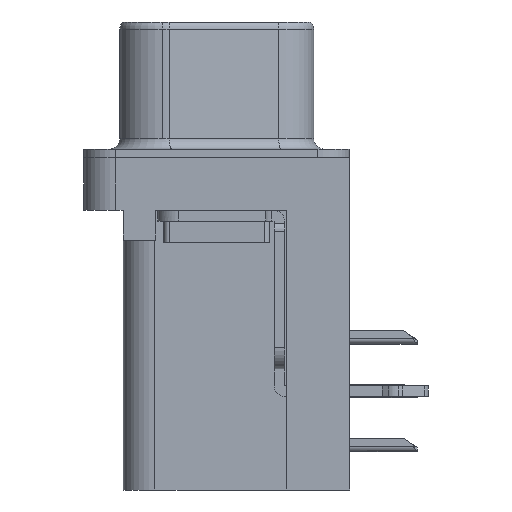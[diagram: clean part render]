
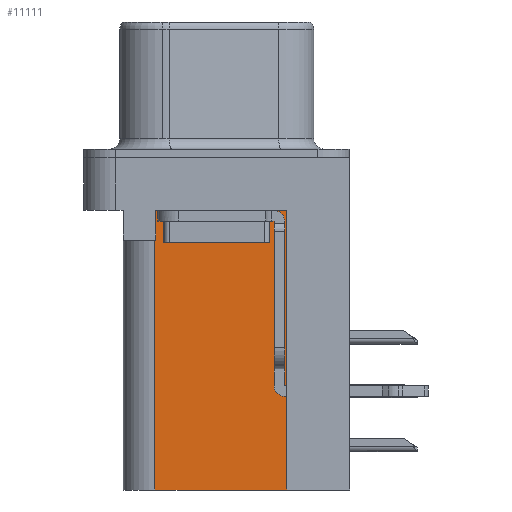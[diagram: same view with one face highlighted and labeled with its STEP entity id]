
A CAD part, left-side view. The second image highlights one B-rep face of the part: STEP entity #11111.
In plain terms, the highlighted planar face has unit normal (-1, 0, 0).
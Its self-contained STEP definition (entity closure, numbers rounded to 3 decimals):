
#153 = PLANE ( 'NONE',  #16543 ) ;
#682 = CARTESIAN_POINT ( 'NONE',  ( 3.765, 2.895, -2.5 ) ) ;
#878 = EDGE_CURVE ( 'NONE', #23352, #19911, #8876, .T. ) ;
#995 = FACE_OUTER_BOUND ( 'NONE', #13016, .T. ) ;
#1602 = DIRECTION ( 'NONE',  ( 0., 0., -1. ) ) ;
#1967 = ORIENTED_EDGE ( 'NONE', *, *, #15726, .F. ) ;
#2036 = LINE ( 'NONE', #19618, #7053 ) ;
#2092 = CARTESIAN_POINT ( 'NONE',  ( 3.765, -3.295, -15.7 ) ) ;
#2804 = DIRECTION ( 'NONE',  ( 0., 1., 0. ) ) ;
#3025 = EDGE_CURVE ( 'NONE', #8518, #22390, #22125, .T. ) ;
#3860 = ORIENTED_EDGE ( 'NONE', *, *, #3025, .F. ) ;
#3994 = DIRECTION ( 'NONE',  ( 1., 0., 0. ) ) ;
#4093 = VECTOR ( 'NONE', #24320, 1000. ) ;
#4317 = EDGE_CURVE ( 'NONE', #8518, #18158, #2036, .T. ) ;
#5150 = ORIENTED_EDGE ( 'NONE', *, *, #4317, .T. ) ;
#5769 = DIRECTION ( 'NONE',  ( 0., 0., 1. ) ) ;
#5838 = VECTOR ( 'NONE', #5769, 1000. ) ;
#6212 = CARTESIAN_POINT ( 'NONE',  ( 3.765, 2.925, -3.9 ) ) ;
#6353 = DIRECTION ( 'NONE',  ( 0., 0., 1. ) ) ;
#6405 = LINE ( 'NONE', #15181, #5838 ) ;
#6591 = EDGE_CURVE ( 'NONE', #18158, #23352, #23307, .T. ) ;
#7053 = VECTOR ( 'NONE', #6353, 1000. ) ;
#8518 = VERTEX_POINT ( 'NONE', #13735 ) ;
#8876 = LINE ( 'NONE', #22612, #13333 ) ;
#9128 = LINE ( 'NONE', #16618, #4093 ) ;
#11111 = ADVANCED_FACE ( 'NONE', ( #995 ), #153, .F. ) ;
#12331 = ORIENTED_EDGE ( 'NONE', *, *, #14864, .T. ) ;
#12446 = VERTEX_POINT ( 'NONE', #6212 ) ;
#12631 = VECTOR ( 'NONE', #23086, 1000. ) ;
#13016 = EDGE_LOOP ( 'NONE', ( #13136, #13579, #12331, #1967, #3860, #5150 ) ) ;
#13136 = ORIENTED_EDGE ( 'NONE', *, *, #6591, .T. ) ;
#13333 = VECTOR ( 'NONE', #1602, 1000. ) ;
#13579 = ORIENTED_EDGE ( 'NONE', *, *, #878, .T. ) ;
#13735 = CARTESIAN_POINT ( 'NONE',  ( 3.765, -3.295, -15.7 ) ) ;
#13740 = CARTESIAN_POINT ( 'NONE',  ( 3.765, -3.295, -2.5 ) ) ;
#13950 = CARTESIAN_POINT ( 'NONE',  ( 3.765, 2.925, -15.7 ) ) ;
#14864 = EDGE_CURVE ( 'NONE', #19911, #12446, #9128, .T. ) ;
#15181 = CARTESIAN_POINT ( 'NONE',  ( 3.765, 2.925, -15.7 ) ) ;
#15726 = EDGE_CURVE ( 'NONE', #22390, #12446, #6405, .T. ) ;
#16543 = AXIS2_PLACEMENT_3D ( 'NONE', #2092, #3994, #17221 ) ;
#16618 = CARTESIAN_POINT ( 'NONE',  ( 3.765, 0., -3.9 ) ) ;
#17221 = DIRECTION ( 'NONE',  ( 0., 0., -1. ) ) ;
#18158 = VERTEX_POINT ( 'NONE', #13740 ) ;
#19355 = CARTESIAN_POINT ( 'NONE',  ( 3.765, -3.295, -15.7 ) ) ;
#19618 = CARTESIAN_POINT ( 'NONE',  ( 3.765, -3.295, -15.7 ) ) ;
#19911 = VERTEX_POINT ( 'NONE', #22280 ) ;
#20958 = VECTOR ( 'NONE', #2804, 1000. ) ;
#21188 = CARTESIAN_POINT ( 'NONE',  ( 3.765, -3.295, -2.5 ) ) ;
#22125 = LINE ( 'NONE', #19355, #20958 ) ;
#22280 = CARTESIAN_POINT ( 'NONE',  ( 3.765, 2.895, -3.9 ) ) ;
#22390 = VERTEX_POINT ( 'NONE', #13950 ) ;
#22612 = CARTESIAN_POINT ( 'NONE',  ( 3.765, 2.895, -3.9 ) ) ;
#23086 = DIRECTION ( 'NONE',  ( 0., 1., 0. ) ) ;
#23307 = LINE ( 'NONE', #21188, #12631 ) ;
#23352 = VERTEX_POINT ( 'NONE', #682 ) ;
#24320 = DIRECTION ( 'NONE',  ( 0., 1., 0. ) ) ;
